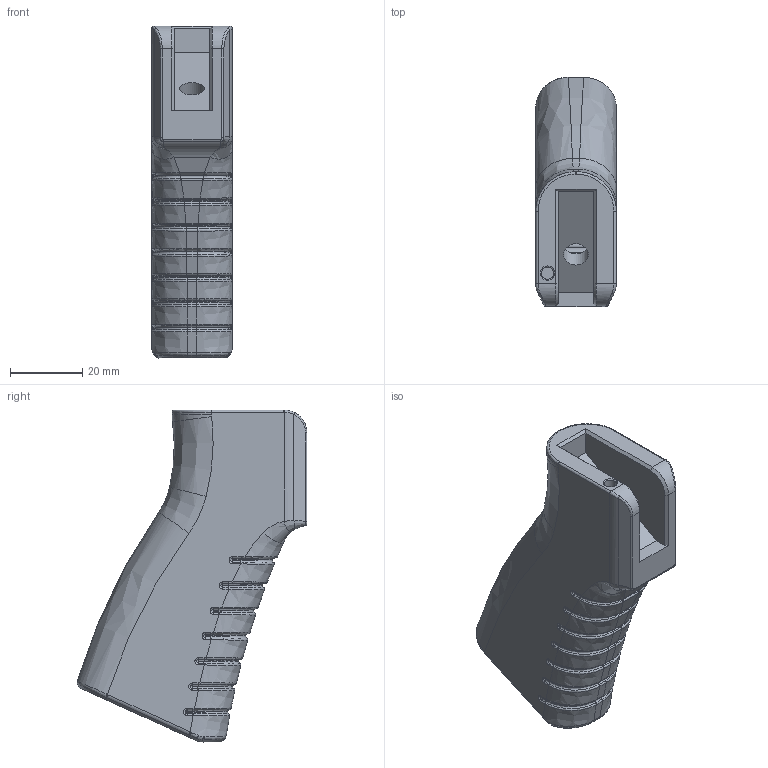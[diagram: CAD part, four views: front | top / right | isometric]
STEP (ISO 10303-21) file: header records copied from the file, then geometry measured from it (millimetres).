
FILE_DESCRIPTION(/* description */ (''),/* implementation_level */ '2;1');
FILE_NAME(/* name */ 'Grip 3.step',/* time_stamp */ '2021-10-28T08:42:53-04:00',/* author */ (''),/* organization */ (''),/* preprocessor_version */ 'ST-DEVELOPER v18.1',/* originating_system */ 'Autodesk Translation Framework v10.10.0.1391',/* authorisation */ '');
FILE_SCHEMA (('AUTOMOTIVE_DESIGN { 1 0 10303 214 3 1 1 }'));
Products named in the file (1): Grip 3
Bounding box: 22.33 x 63.64 x 91.97 mm (x, y, z)
Volume: 39476.7 mm3; surface area: 18086.6 mm2
Topology: 1 solids, 1 shells, 942 faces, 2389 edges, 1439 vertices
Faces by surface type: bspline 583, cylinder 186, plane 85, torus 81, cone 7
Full cylindrical faces by diameter (mm): 3.4 x1, 6.8 x1, 11.616 x1, 13.416 x1
Entity records: 45573 total; most frequent: CARTESIAN_POINT 26366, ORIENTED_EDGE 4730, DIRECTION 2789, EDGE_CURVE 2365, VERTEX_POINT 1439, AXIS2_PLACEMENT_3D 1058, B_SPLINE_CURVE_WITH_KNOTS 994, EDGE_LOOP 958
